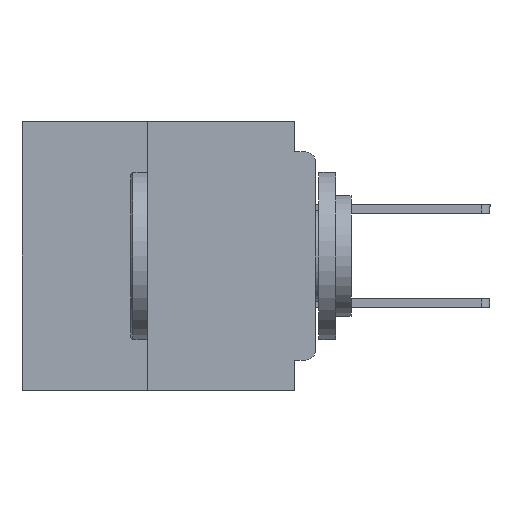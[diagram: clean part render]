
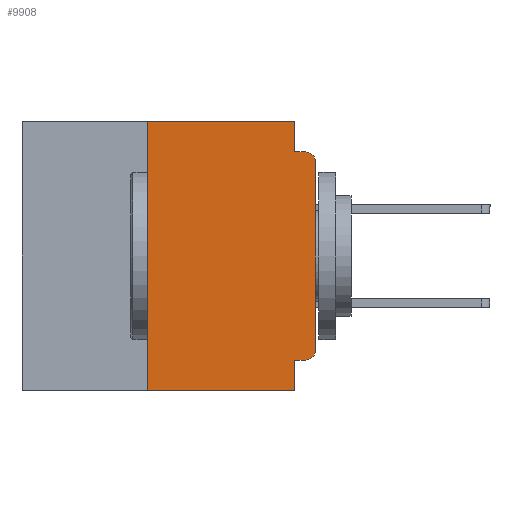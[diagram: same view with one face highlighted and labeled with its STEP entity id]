
A CAD part, left-side view. The second image highlights one B-rep face of the part: STEP entity #9908.
In plain terms, the highlighted planar face has unit normal (-1, 0, 0).
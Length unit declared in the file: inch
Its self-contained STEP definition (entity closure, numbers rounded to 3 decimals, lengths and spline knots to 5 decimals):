
#114 = DIRECTION ( 'NONE',  ( 0., 0., -1. ) ) ;
#275 = VERTEX_POINT ( 'NONE', #29110 ) ;
#330 = EDGE_CURVE ( 'NONE', #33823, #43858, #27197, .T. ) ;
#388 = AXIS2_PLACEMENT_3D ( 'NONE', #12785, #36798, #16239 ) ;
#651 = CARTESIAN_POINT ( 'NONE',  ( 0., 0.437, -0.4 ) ) ;
#905 = VECTOR ( 'NONE', #11345, 39.37008 ) ;
#1379 = EDGE_CURVE ( 'NONE', #37250, #42453, #3446, .T. ) ;
#1441 = CIRCLE ( 'NONE', #388, 0.015 ) ;
#3056 = CARTESIAN_POINT ( 'NONE',  ( 0., 0.25, 0. ) ) ;
#3275 = CARTESIAN_POINT ( 'NONE',  ( 0., 0., -0.34 ) ) ;
#3440 = VECTOR ( 'NONE', #35155, 39.37008 ) ;
#3446 = CIRCLE ( 'NONE', #18493, 0.015 ) ;
#3729 = CARTESIAN_POINT ( 'NONE',  ( 0., 0.031, -0.045 ) ) ;
#3894 = ORIENTED_EDGE ( 'NONE', *, *, #30030, .F. ) ;
#4661 = DIRECTION ( 'NONE',  ( 0., 0., 1. ) ) ;
#5408 = LINE ( 'NONE', #651, #40781 ) ;
#5636 = EDGE_LOOP ( 'NONE', ( #43229, #11607, #16677, #19565, #28569, #3894, #33629, #34783, #29027, #31271 ) ) ;
#6249 = VERTEX_POINT ( 'NONE', #3056 ) ;
#7837 = VECTOR ( 'NONE', #12784, 39.37008 ) ;
#8868 = VECTOR ( 'NONE', #4661, 39.37008 ) ;
#9908 = ADVANCED_FACE ( 'NONE', ( #28177 ), #37777, .F. ) ;
#10001 = LINE ( 'NONE', #28455, #905 ) ;
#11184 = CARTESIAN_POINT ( 'NONE',  ( 0., 0.015, -0.06 ) ) ;
#11194 = DIRECTION ( 'NONE',  ( -1., 0., 0. ) ) ;
#11201 = VERTEX_POINT ( 'NONE', #34075 ) ;
#11281 = DIRECTION ( 'NONE',  ( 0., 0., -1. ) ) ;
#11345 = DIRECTION ( 'NONE',  ( 0., -1., 0. ) ) ;
#11424 = DIRECTION ( 'NONE',  ( 0., 1., 0. ) ) ;
#11607 = ORIENTED_EDGE ( 'NONE', *, *, #1379, .T. ) ;
#12562 = LINE ( 'NONE', #35006, #3440 ) ;
#12784 = DIRECTION ( 'NONE',  ( 0., 0., -1. ) ) ;
#12785 = CARTESIAN_POINT ( 'NONE',  ( 0., 0.015, -0.34 ) ) ;
#14432 = DIRECTION ( 'NONE',  ( 0., -1., 0. ) ) ;
#15029 = EDGE_CURVE ( 'NONE', #275, #43793, #1441, .T. ) ;
#15714 = VECTOR ( 'NONE', #19643, 39.37008 ) ;
#16239 = DIRECTION ( 'NONE',  ( 0., 0., -1. ) ) ;
#16573 = AXIS2_PLACEMENT_3D ( 'NONE', #17195, #20635, #114 ) ;
#16677 = ORIENTED_EDGE ( 'NONE', *, *, #19814, .F. ) ;
#16787 = LINE ( 'NONE', #36937, #15714 ) ;
#17195 = CARTESIAN_POINT ( 'NONE',  ( 0., 0.437, 0. ) ) ;
#18376 = EDGE_CURVE ( 'NONE', #20726, #11201, #37001, .T. ) ;
#18493 = AXIS2_PLACEMENT_3D ( 'NONE', #11184, #11194, #11281 ) ;
#19565 = ORIENTED_EDGE ( 'NONE', *, *, #330, .F. ) ;
#19643 = DIRECTION ( 'NONE',  ( 0., -1., 0. ) ) ;
#19646 = DIRECTION ( 'NONE',  ( 0., 0., -1. ) ) ;
#19814 = EDGE_CURVE ( 'NONE', #43858, #42453, #10001, .T. ) ;
#20097 = VERTEX_POINT ( 'NONE', #36796 ) ;
#20635 = DIRECTION ( 'NONE',  ( 1., 0., 0. ) ) ;
#20717 = VECTOR ( 'NONE', #11424, 39.37008 ) ;
#20726 = VERTEX_POINT ( 'NONE', #23083 ) ;
#23083 = CARTESIAN_POINT ( 'NONE',  ( 0., 0.031, -0.355 ) ) ;
#25981 = EDGE_CURVE ( 'NONE', #43793, #37250, #12562, .T. ) ;
#26822 = VECTOR ( 'NONE', #19646, 39.37008 ) ;
#27197 = LINE ( 'NONE', #27607, #7837 ) ;
#27607 = CARTESIAN_POINT ( 'NONE',  ( 0., 0.031, 0. ) ) ;
#27864 = CARTESIAN_POINT ( 'NONE',  ( 0., 0., -0.06 ) ) ;
#28177 = FACE_OUTER_BOUND ( 'NONE', #5636, .T. ) ;
#28455 = CARTESIAN_POINT ( 'NONE',  ( 0., 0., -0.045 ) ) ;
#28569 = ORIENTED_EDGE ( 'NONE', *, *, #31436, .F. ) ;
#29027 = ORIENTED_EDGE ( 'NONE', *, *, #33395, .F. ) ;
#29110 = CARTESIAN_POINT ( 'NONE',  ( 0., 0.015, -0.355 ) ) ;
#29862 = LINE ( 'NONE', #42090, #20717 ) ;
#30030 = EDGE_CURVE ( 'NONE', #20097, #6249, #36259, .T. ) ;
#30045 = CARTESIAN_POINT ( 'NONE',  ( 0., 0.031, -0.4 ) ) ;
#31271 = ORIENTED_EDGE ( 'NONE', *, *, #15029, .T. ) ;
#31436 = EDGE_CURVE ( 'NONE', #6249, #33823, #16787, .T. ) ;
#33395 = EDGE_CURVE ( 'NONE', #275, #20726, #29862, .T. ) ;
#33629 = ORIENTED_EDGE ( 'NONE', *, *, #40683, .T. ) ;
#33823 = VERTEX_POINT ( 'NONE', #34188 ) ;
#34075 = CARTESIAN_POINT ( 'NONE',  ( 0., 0.031, -0.4 ) ) ;
#34188 = CARTESIAN_POINT ( 'NONE',  ( 0., 0.031, 0. ) ) ;
#34783 = ORIENTED_EDGE ( 'NONE', *, *, #18376, .F. ) ;
#35006 = CARTESIAN_POINT ( 'NONE',  ( 0., 0., 0. ) ) ;
#35155 = DIRECTION ( 'NONE',  ( 0., 0., 1. ) ) ;
#35547 = CARTESIAN_POINT ( 'NONE',  ( 0., 0.25, -0.4 ) ) ;
#36259 = LINE ( 'NONE', #35547, #8868 ) ;
#36796 = CARTESIAN_POINT ( 'NONE',  ( 0., 0.25, -0.4 ) ) ;
#36798 = DIRECTION ( 'NONE',  ( -1., 0., 0. ) ) ;
#36937 = CARTESIAN_POINT ( 'NONE',  ( 0., 0.437, 0. ) ) ;
#37001 = LINE ( 'NONE', #30045, #26822 ) ;
#37250 = VERTEX_POINT ( 'NONE', #27864 ) ;
#37777 = PLANE ( 'NONE',  #16573 ) ;
#40254 = CARTESIAN_POINT ( 'NONE',  ( 0., 0.015, -0.045 ) ) ;
#40683 = EDGE_CURVE ( 'NONE', #20097, #11201, #5408, .T. ) ;
#40781 = VECTOR ( 'NONE', #14432, 39.37008 ) ;
#42090 = CARTESIAN_POINT ( 'NONE',  ( 0., 0., -0.355 ) ) ;
#42453 = VERTEX_POINT ( 'NONE', #40254 ) ;
#43229 = ORIENTED_EDGE ( 'NONE', *, *, #25981, .T. ) ;
#43793 = VERTEX_POINT ( 'NONE', #3275 ) ;
#43858 = VERTEX_POINT ( 'NONE', #3729 ) ;
